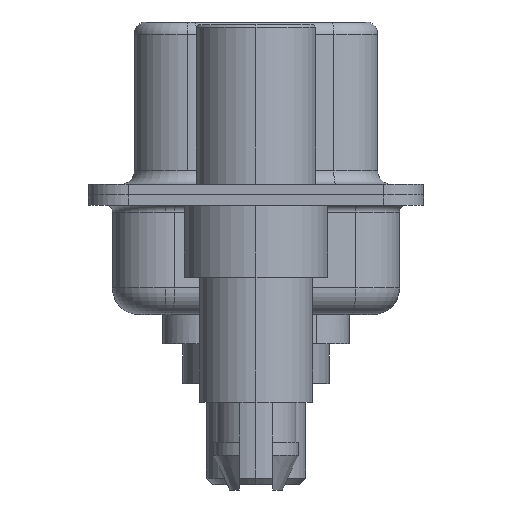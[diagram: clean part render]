
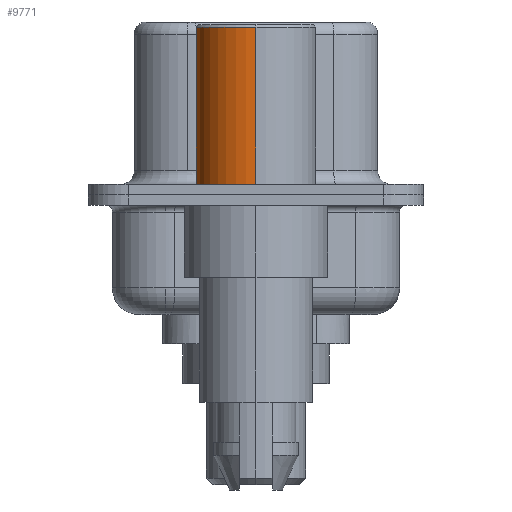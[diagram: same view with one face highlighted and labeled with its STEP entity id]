
A CAD part, left-side view. The second image highlights one B-rep face of the part: STEP entity #9771.
In plain terms, the highlighted cylindrical face has radius 2.25 mm (diameter 4.5 mm), a partial arc.
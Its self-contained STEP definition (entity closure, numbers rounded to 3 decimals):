
#272 = EDGE_CURVE ( 'NONE', #15541, #12682, #13532, .T. ) ;
#654 = EDGE_CURVE ( 'NONE', #12055, #12682, #7984, .T. ) ;
#1057 = CYLINDRICAL_SURFACE ( 'NONE', #11632, 2.25 ) ;
#1191 = CARTESIAN_POINT ( 'NONE',  ( 2.25, 0., 6.3 ) ) ;
#1341 = VECTOR ( 'NONE', #9403, 1000. ) ;
#1821 = EDGE_CURVE ( 'NONE', #18217, #15541, #4268, .T. ) ;
#3065 = DIRECTION ( 'NONE',  ( 0., 0., 1. ) ) ;
#4218 = ORIENTED_EDGE ( 'NONE', *, *, #272, .T. ) ;
#4268 = CIRCLE ( 'NONE', #18487, 2.25 ) ;
#4974 = DIRECTION ( 'NONE',  ( 1., 0., 0. ) ) ;
#5145 = DIRECTION ( 'NONE',  ( 0., 0., 1. ) ) ;
#5154 = AXIS2_PLACEMENT_3D ( 'NONE', #6161, #5145, #4974 ) ;
#5181 = ORIENTED_EDGE ( 'NONE', *, *, #13403, .F. ) ;
#5200 = ORIENTED_EDGE ( 'NONE', *, *, #1821, .T. ) ;
#6161 = CARTESIAN_POINT ( 'NONE',  ( 0., 0., 6.3 ) ) ;
#6252 = DIRECTION ( 'NONE',  ( 1., 0., 0. ) ) ;
#6397 = DIRECTION ( 'NONE',  ( 0., 0., 1. ) ) ;
#7179 = DIRECTION ( 'NONE',  ( 1., 0., 0. ) ) ;
#7318 = CARTESIAN_POINT ( 'NONE',  ( 0., 0., 0.4 ) ) ;
#7984 = CIRCLE ( 'NONE', #5154, 2.25 ) ;
#8393 = CARTESIAN_POINT ( 'NONE',  ( -2.25, 0., 0.4 ) ) ;
#8635 = DIRECTION ( 'NONE',  ( 0., 0., 1. ) ) ;
#9382 = CARTESIAN_POINT ( 'NONE',  ( -2.25, 0., 0.581 ) ) ;
#9403 = DIRECTION ( 'NONE',  ( 0., 0., 1. ) ) ;
#9771 = ADVANCED_FACE ( 'NONE', ( #12798 ), #1057, .T. ) ;
#11069 = CARTESIAN_POINT ( 'NONE',  ( 2.25, 0., 0.4 ) ) ;
#11632 = AXIS2_PLACEMENT_3D ( 'NONE', #17449, #8635, #7179 ) ;
#12055 = VERTEX_POINT ( 'NONE', #1191 ) ;
#12682 = VERTEX_POINT ( 'NONE', #17441 ) ;
#12798 = FACE_OUTER_BOUND ( 'NONE', #18570, .T. ) ;
#13403 = EDGE_CURVE ( 'NONE', #18217, #12055, #18694, .T. ) ;
#13532 = LINE ( 'NONE', #9382, #1341 ) ;
#14255 = VECTOR ( 'NONE', #3065, 1000. ) ;
#14650 = ORIENTED_EDGE ( 'NONE', *, *, #654, .F. ) ;
#14827 = CARTESIAN_POINT ( 'NONE',  ( 2.25, 0., 0.581 ) ) ;
#15541 = VERTEX_POINT ( 'NONE', #8393 ) ;
#17441 = CARTESIAN_POINT ( 'NONE',  ( -2.25, 0., 6.3 ) ) ;
#17449 = CARTESIAN_POINT ( 'NONE',  ( 0., 0., 0.581 ) ) ;
#18217 = VERTEX_POINT ( 'NONE', #11069 ) ;
#18487 = AXIS2_PLACEMENT_3D ( 'NONE', #7318, #6397, #6252 ) ;
#18570 = EDGE_LOOP ( 'NONE', ( #5200, #4218, #14650, #5181 ) ) ;
#18694 = LINE ( 'NONE', #14827, #14255 ) ;
